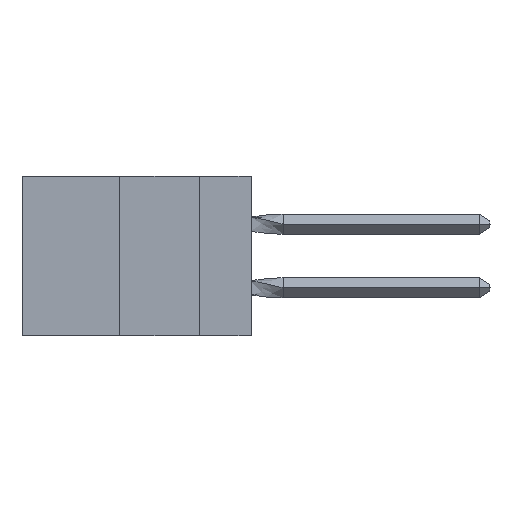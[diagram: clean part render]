
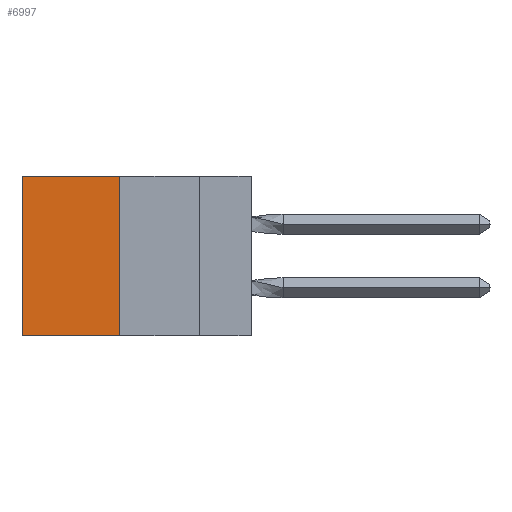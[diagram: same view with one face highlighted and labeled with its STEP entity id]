
A CAD part, left-side view. The second image highlights one B-rep face of the part: STEP entity #6997.
In plain terms, the highlighted planar face has unit normal (-1, 0, 0).
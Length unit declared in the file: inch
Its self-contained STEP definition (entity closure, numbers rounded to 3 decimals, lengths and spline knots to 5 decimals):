
#554 = ORIENTED_EDGE ( 'NONE', *, *, #27175, .T. ) ;
#604 = LINE ( 'NONE', #18548, #14960 ) ;
#2724 = CARTESIAN_POINT ( 'NONE',  ( 0.305, 0.413, 0. ) ) ;
#4018 = ORIENTED_EDGE ( 'NONE', *, *, #24219, .T. ) ;
#4610 = VERTEX_POINT ( 'NONE', #5617 ) ;
#4669 = LINE ( 'NONE', #2724, #17184 ) ;
#5504 = PLANE ( 'NONE',  #16686 ) ;
#5617 = CARTESIAN_POINT ( 'NONE',  ( 0.305, 0.413, 0. ) ) ;
#5701 = EDGE_CURVE ( 'NONE', #4610, #10375, #604, .T. ) ;
#6997 = ADVANCED_FACE ( 'NONE', ( #9113 ), #5504, .F. ) ;
#7754 = CARTESIAN_POINT ( 'NONE',  ( 0.305, 0.413, -0.5 ) ) ;
#8499 = CARTESIAN_POINT ( 'NONE',  ( 0.305, 0.72, -0.5 ) ) ;
#9113 = FACE_OUTER_BOUND ( 'NONE', #24635, .T. ) ;
#9126 = LINE ( 'NONE', #27339, #12053 ) ;
#10375 = VERTEX_POINT ( 'NONE', #18844 ) ;
#11827 = DIRECTION ( 'NONE',  ( 0., 1., 0. ) ) ;
#12053 = VECTOR ( 'NONE', #16520, 39.37008 ) ;
#13067 = CARTESIAN_POINT ( 'NONE',  ( 0.305, 0.72, 0. ) ) ;
#13510 = VERTEX_POINT ( 'NONE', #8499 ) ;
#14594 = DIRECTION ( 'NONE',  ( 1., 0., 0. ) ) ;
#14690 = DIRECTION ( 'NONE',  ( 0., 1., 0. ) ) ;
#14960 = VECTOR ( 'NONE', #18856, 39.37008 ) ;
#16520 = DIRECTION ( 'NONE',  ( 0., 0., -1. ) ) ;
#16660 = CARTESIAN_POINT ( 'NONE',  ( 0.305, 0.413, -0.5 ) ) ;
#16686 = AXIS2_PLACEMENT_3D ( 'NONE', #7754, #14594, #24030 ) ;
#17001 = ORIENTED_EDGE ( 'NONE', *, *, #5701, .F. ) ;
#17184 = VECTOR ( 'NONE', #11827, 39.37008 ) ;
#18548 = CARTESIAN_POINT ( 'NONE',  ( 0.305, 0.413, -0.5 ) ) ;
#18799 = LINE ( 'NONE', #16660, #25216 ) ;
#18844 = CARTESIAN_POINT ( 'NONE',  ( 0.305, 0.413, -0.5 ) ) ;
#18856 = DIRECTION ( 'NONE',  ( 0., 0., -1. ) ) ;
#20018 = VERTEX_POINT ( 'NONE', #13067 ) ;
#22394 = ORIENTED_EDGE ( 'NONE', *, *, #23862, .F. ) ;
#23862 = EDGE_CURVE ( 'NONE', #10375, #13510, #18799, .T. ) ;
#24030 = DIRECTION ( 'NONE',  ( 0., 0., -1. ) ) ;
#24219 = EDGE_CURVE ( 'NONE', #20018, #13510, #9126, .T. ) ;
#24635 = EDGE_LOOP ( 'NONE', ( #4018, #22394, #17001, #554 ) ) ;
#25216 = VECTOR ( 'NONE', #14690, 39.37008 ) ;
#27175 = EDGE_CURVE ( 'NONE', #4610, #20018, #4669, .T. ) ;
#27339 = CARTESIAN_POINT ( 'NONE',  ( 0.305, 0.72, -0.5 ) ) ;
